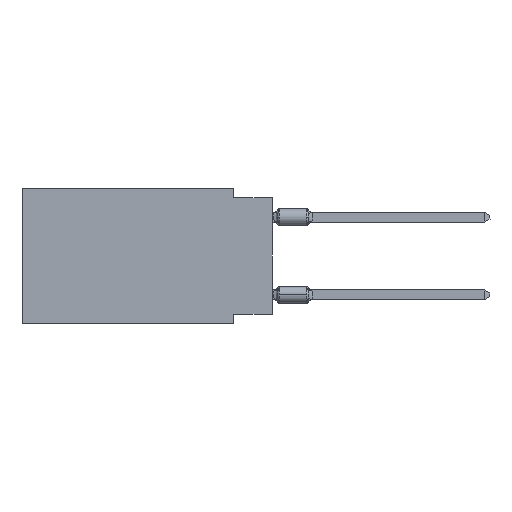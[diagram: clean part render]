
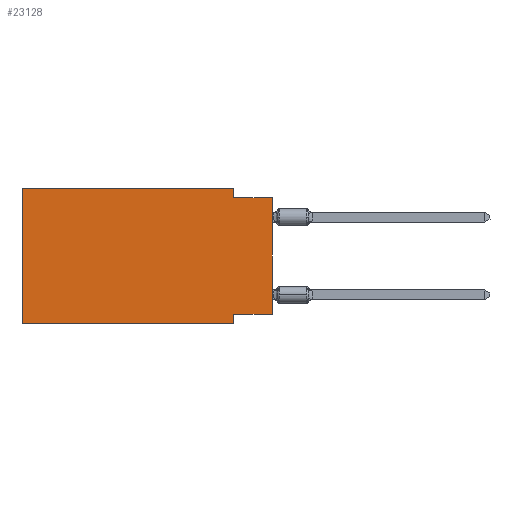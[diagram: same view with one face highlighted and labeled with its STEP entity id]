
A CAD part, left-side view. The second image highlights one B-rep face of the part: STEP entity #23128.
In plain terms, the highlighted planar face has unit normal (-1, 0, 0).
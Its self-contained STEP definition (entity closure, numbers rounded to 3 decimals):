
#688 = DIRECTION ( 'NONE',  ( 0., 0., 1. ) ) ;
#973 = EDGE_CURVE ( 'NONE', #2449, #19490, #19186, .T. ) ;
#1447 = DIRECTION ( 'NONE',  ( 0., -1., 0. ) ) ;
#1480 = VERTEX_POINT ( 'NONE', #28579 ) ;
#1924 = LINE ( 'NONE', #23351, #3959 ) ;
#1975 = ORIENTED_EDGE ( 'NONE', *, *, #10204, .T. ) ;
#2449 = VERTEX_POINT ( 'NONE', #13321 ) ;
#3162 = VECTOR ( 'NONE', #12563, 1000. ) ;
#3318 = CARTESIAN_POINT ( 'NONE',  ( 0., 0., -8.255 ) ) ;
#3333 = CARTESIAN_POINT ( 'NONE',  ( 0., 16.383, -8.89 ) ) ;
#3959 = VECTOR ( 'NONE', #22742, 1000. ) ;
#4015 = VECTOR ( 'NONE', #23431, 1000. ) ;
#4139 = CARTESIAN_POINT ( 'NONE',  ( 0., 2.54, 0. ) ) ;
#4233 = VECTOR ( 'NONE', #19549, 1000. ) ;
#5082 = LINE ( 'NONE', #4139, #25728 ) ;
#5994 = VERTEX_POINT ( 'NONE', #17966 ) ;
#6310 = DIRECTION ( 'NONE',  ( 0., 0., -1. ) ) ;
#7642 = LINE ( 'NONE', #3318, #3162 ) ;
#8056 = DIRECTION ( 'NONE',  ( 0., 0., -1. ) ) ;
#8551 = LINE ( 'NONE', #15487, #11038 ) ;
#9563 = EDGE_LOOP ( 'NONE', ( #28271, #16523, #20182, #10911, #26644, #1975, #19505, #24894 ) ) ;
#9843 = CARTESIAN_POINT ( 'NONE',  ( 0., 0., 0. ) ) ;
#10204 = EDGE_CURVE ( 'NONE', #2449, #1480, #20121, .T. ) ;
#10911 = ORIENTED_EDGE ( 'NONE', *, *, #16533, .F. ) ;
#11038 = VECTOR ( 'NONE', #1447, 1000. ) ;
#12259 = VERTEX_POINT ( 'NONE', #30345 ) ;
#12563 = DIRECTION ( 'NONE',  ( 0., 1., 0. ) ) ;
#12733 = DIRECTION ( 'NONE',  ( 0., -1., 0. ) ) ;
#13321 = CARTESIAN_POINT ( 'NONE',  ( 0., 16.383, -8.89 ) ) ;
#14703 = CARTESIAN_POINT ( 'NONE',  ( 0., 16.383, 0. ) ) ;
#14852 = PLANE ( 'NONE',  #29866 ) ;
#15487 = CARTESIAN_POINT ( 'NONE',  ( 0., 0., -0.635 ) ) ;
#15634 = EDGE_CURVE ( 'NONE', #28644, #1480, #30218, .T. ) ;
#16523 = ORIENTED_EDGE ( 'NONE', *, *, #21549, .F. ) ;
#16533 = EDGE_CURVE ( 'NONE', #19490, #5994, #1924, .T. ) ;
#17615 = FACE_OUTER_BOUND ( 'NONE', #9563, .T. ) ;
#17966 = CARTESIAN_POINT ( 'NONE',  ( 0., 2.54, 0. ) ) ;
#19186 = LINE ( 'NONE', #26912, #19898 ) ;
#19490 = VERTEX_POINT ( 'NONE', #20181 ) ;
#19505 = ORIENTED_EDGE ( 'NONE', *, *, #15634, .F. ) ;
#19549 = DIRECTION ( 'NONE',  ( 0., 0., 1. ) ) ;
#19898 = VECTOR ( 'NONE', #688, 1000. ) ;
#19938 = VERTEX_POINT ( 'NONE', #27092 ) ;
#20121 = LINE ( 'NONE', #3333, #22559 ) ;
#20181 = CARTESIAN_POINT ( 'NONE',  ( 0., 16.383, 0. ) ) ;
#20182 = ORIENTED_EDGE ( 'NONE', *, *, #29005, .F. ) ;
#21494 = EDGE_CURVE ( 'NONE', #24719, #28644, #7642, .T. ) ;
#21549 = EDGE_CURVE ( 'NONE', #19938, #12259, #8551, .T. ) ;
#22559 = VECTOR ( 'NONE', #12733, 1000. ) ;
#22670 = EDGE_CURVE ( 'NONE', #24719, #12259, #26057, .T. ) ;
#22742 = DIRECTION ( 'NONE',  ( 0., -1., 0. ) ) ;
#22976 = CARTESIAN_POINT ( 'NONE',  ( 0., 2.54, -8.89 ) ) ;
#23128 = ADVANCED_FACE ( 'NONE', ( #17615 ), #14852, .F. ) ;
#23351 = CARTESIAN_POINT ( 'NONE',  ( 0., 16.383, 0. ) ) ;
#23431 = DIRECTION ( 'NONE',  ( 0., 0., -1. ) ) ;
#24719 = VERTEX_POINT ( 'NONE', #24995 ) ;
#24894 = ORIENTED_EDGE ( 'NONE', *, *, #21494, .F. ) ;
#24995 = CARTESIAN_POINT ( 'NONE',  ( 0., 0., -8.255 ) ) ;
#25728 = VECTOR ( 'NONE', #6310, 1000. ) ;
#26057 = LINE ( 'NONE', #9843, #4233 ) ;
#26644 = ORIENTED_EDGE ( 'NONE', *, *, #973, .F. ) ;
#26912 = CARTESIAN_POINT ( 'NONE',  ( 0., 16.383, 0. ) ) ;
#27092 = CARTESIAN_POINT ( 'NONE',  ( 0., 2.54, -0.635 ) ) ;
#28271 = ORIENTED_EDGE ( 'NONE', *, *, #22670, .T. ) ;
#28579 = CARTESIAN_POINT ( 'NONE',  ( 0., 2.54, -8.89 ) ) ;
#28644 = VERTEX_POINT ( 'NONE', #29629 ) ;
#28900 = DIRECTION ( 'NONE',  ( 1., 0., 0. ) ) ;
#29005 = EDGE_CURVE ( 'NONE', #5994, #19938, #5082, .T. ) ;
#29629 = CARTESIAN_POINT ( 'NONE',  ( 0., 2.54, -8.255 ) ) ;
#29866 = AXIS2_PLACEMENT_3D ( 'NONE', #14703, #28900, #8056 ) ;
#30218 = LINE ( 'NONE', #22976, #4015 ) ;
#30345 = CARTESIAN_POINT ( 'NONE',  ( 0., 0., -0.635 ) ) ;
